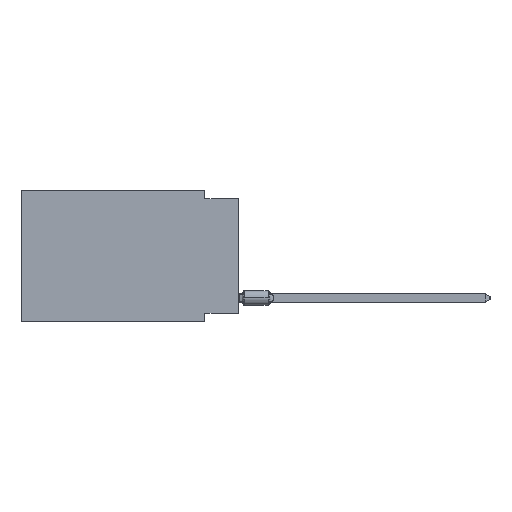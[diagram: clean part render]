
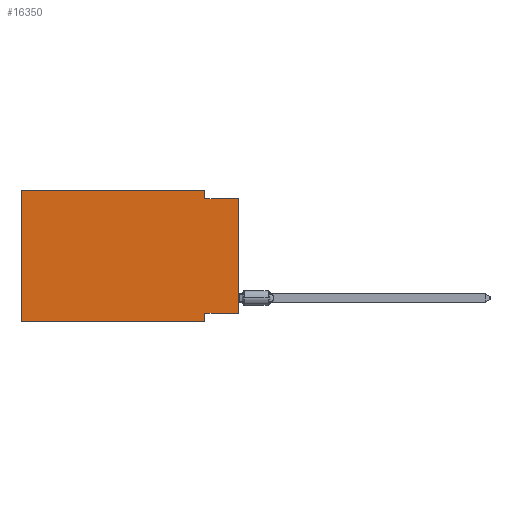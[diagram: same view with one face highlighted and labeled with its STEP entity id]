
A CAD part, left-side view. The second image highlights one B-rep face of the part: STEP entity #16350.
In plain terms, the highlighted planar face has unit normal (-1, 0, 0).
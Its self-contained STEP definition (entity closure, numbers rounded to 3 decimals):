
#1029 = VERTEX_POINT ( 'NONE', #79012 ) ;
#1121 = CARTESIAN_POINT ( 'NONE',  ( 0., 2.54, -9.906 ) ) ;
#1714 = VERTEX_POINT ( 'NONE', #8603 ) ;
#2498 = VERTEX_POINT ( 'NONE', #78590 ) ;
#3478 = VECTOR ( 'NONE', #12910, 1000. ) ;
#4124 = EDGE_CURVE ( 'NONE', #28901, #12446, #36039, .T. ) ;
#4131 = ORIENTED_EDGE ( 'NONE', *, *, #31196, .T. ) ;
#4492 = DIRECTION ( 'NONE',  ( 0., -1., 0. ) ) ;
#4829 = PLANE ( 'NONE',  #26625 ) ;
#7272 = EDGE_CURVE ( 'NONE', #29020, #1714, #59118, .T. ) ;
#7627 = DIRECTION ( 'NONE',  ( 0., 0., -1. ) ) ;
#8603 = CARTESIAN_POINT ( 'NONE',  ( 0., 2.54, -0.635 ) ) ;
#12446 = VERTEX_POINT ( 'NONE', #60024 ) ;
#12910 = DIRECTION ( 'NONE',  ( 0., 0., 1. ) ) ;
#13795 = CARTESIAN_POINT ( 'NONE',  ( 0., 0., -0.635 ) ) ;
#16350 = ADVANCED_FACE ( 'NONE', ( #73460 ), #4829, .F. ) ;
#19548 = LINE ( 'NONE', #31470, #51796 ) ;
#21792 = ORIENTED_EDGE ( 'NONE', *, *, #53097, .F. ) ;
#22599 = LINE ( 'NONE', #66142, #57034 ) ;
#23830 = DIRECTION ( 'NONE',  ( 0., 0., 1. ) ) ;
#26625 = AXIS2_PLACEMENT_3D ( 'NONE', #54946, #68501, #29894 ) ;
#26922 = ORIENTED_EDGE ( 'NONE', *, *, #4124, .F. ) ;
#28901 = VERTEX_POINT ( 'NONE', #40520 ) ;
#29020 = VERTEX_POINT ( 'NONE', #37601 ) ;
#29050 = DIRECTION ( 'NONE',  ( 0., 1., 0. ) ) ;
#29894 = DIRECTION ( 'NONE',  ( 0., 0., -1. ) ) ;
#30755 = ORIENTED_EDGE ( 'NONE', *, *, #35047, .F. ) ;
#31185 = LINE ( 'NONE', #80095, #40554 ) ;
#31196 = EDGE_CURVE ( 'NONE', #1029, #61964, #22599, .T. ) ;
#31470 = CARTESIAN_POINT ( 'NONE',  ( 0., 2.54, -9.906 ) ) ;
#33043 = LINE ( 'NONE', #69219, #3478 ) ;
#33352 = EDGE_CURVE ( 'NONE', #1029, #64289, #33043, .T. ) ;
#34604 = EDGE_LOOP ( 'NONE', ( #77732, #30755, #63373, #39455, #63445, #4131, #21792, #26922 ) ) ;
#35047 = EDGE_CURVE ( 'NONE', #1714, #2498, #76668, .T. ) ;
#35775 = EDGE_CURVE ( 'NONE', #28901, #2498, #31185, .T. ) ;
#36039 = LINE ( 'NONE', #48753, #78405 ) ;
#37601 = CARTESIAN_POINT ( 'NONE',  ( 0., 2.54, 0. ) ) ;
#39455 = ORIENTED_EDGE ( 'NONE', *, *, #53830, .F. ) ;
#40520 = CARTESIAN_POINT ( 'NONE',  ( 0., 0., -9.271 ) ) ;
#40554 = VECTOR ( 'NONE', #23830, 1000. ) ;
#43026 = VECTOR ( 'NONE', #45035, 1000. ) ;
#45035 = DIRECTION ( 'NONE',  ( 0., -1., 0. ) ) ;
#46368 = DIRECTION ( 'NONE',  ( 0., 0., -1. ) ) ;
#47738 = DIRECTION ( 'NONE',  ( 0., -1., 0. ) ) ;
#48753 = CARTESIAN_POINT ( 'NONE',  ( 0., 0., -9.271 ) ) ;
#51796 = VECTOR ( 'NONE', #7627, 1000. ) ;
#52340 = VECTOR ( 'NONE', #46368, 1000. ) ;
#53097 = EDGE_CURVE ( 'NONE', #12446, #61964, #19548, .T. ) ;
#53830 = EDGE_CURVE ( 'NONE', #64289, #29020, #67854, .T. ) ;
#54946 = CARTESIAN_POINT ( 'NONE',  ( 0., 16.383, 0. ) ) ;
#55024 = CARTESIAN_POINT ( 'NONE',  ( 0., 16.383, 0. ) ) ;
#57034 = VECTOR ( 'NONE', #4492, 1000. ) ;
#59118 = LINE ( 'NONE', #77226, #52340 ) ;
#60024 = CARTESIAN_POINT ( 'NONE',  ( 0., 2.54, -9.271 ) ) ;
#61964 = VERTEX_POINT ( 'NONE', #1121 ) ;
#63373 = ORIENTED_EDGE ( 'NONE', *, *, #7272, .F. ) ;
#63445 = ORIENTED_EDGE ( 'NONE', *, *, #33352, .F. ) ;
#64289 = VERTEX_POINT ( 'NONE', #55024 ) ;
#66142 = CARTESIAN_POINT ( 'NONE',  ( 0., 16.383, -9.906 ) ) ;
#67854 = LINE ( 'NONE', #78963, #76874 ) ;
#68501 = DIRECTION ( 'NONE',  ( 1., 0., 0. ) ) ;
#69219 = CARTESIAN_POINT ( 'NONE',  ( 0., 16.383, 0. ) ) ;
#73460 = FACE_OUTER_BOUND ( 'NONE', #34604, .T. ) ;
#76668 = LINE ( 'NONE', #13795, #43026 ) ;
#76874 = VECTOR ( 'NONE', #47738, 1000. ) ;
#77226 = CARTESIAN_POINT ( 'NONE',  ( 0., 2.54, 0. ) ) ;
#77732 = ORIENTED_EDGE ( 'NONE', *, *, #35775, .T. ) ;
#78405 = VECTOR ( 'NONE', #29050, 1000. ) ;
#78590 = CARTESIAN_POINT ( 'NONE',  ( 0., 0., -0.635 ) ) ;
#78963 = CARTESIAN_POINT ( 'NONE',  ( 0., 16.383, 0. ) ) ;
#79012 = CARTESIAN_POINT ( 'NONE',  ( 0., 16.383, -9.906 ) ) ;
#80095 = CARTESIAN_POINT ( 'NONE',  ( 0., 0., 0. ) ) ;
